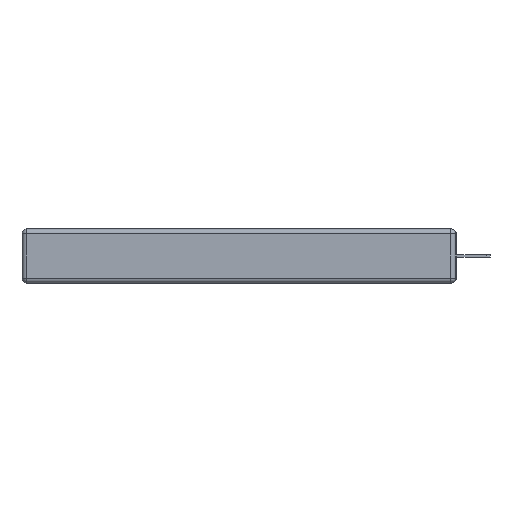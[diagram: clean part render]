
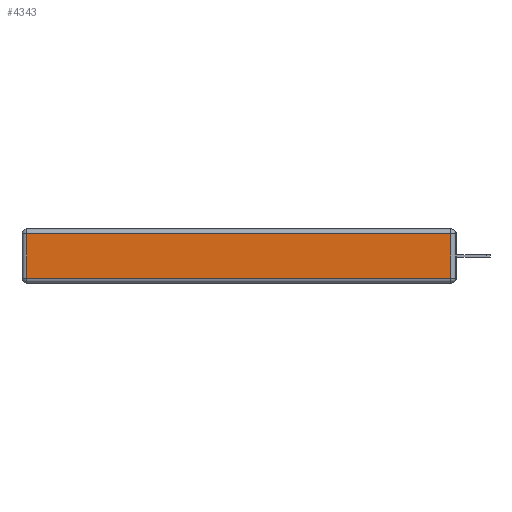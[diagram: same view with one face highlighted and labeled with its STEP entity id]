
A CAD part, left-side view. The second image highlights one B-rep face of the part: STEP entity #4343.
In plain terms, the highlighted planar face has unit normal (-1, 0, 0).
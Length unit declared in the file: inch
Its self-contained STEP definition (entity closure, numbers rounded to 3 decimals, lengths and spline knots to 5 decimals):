
#476 = ORIENTED_EDGE ( 'NONE', *, *, #2474, .T. ) ;
#554 = CARTESIAN_POINT ( 'NONE',  ( 0., 2.72, -0.313 ) ) ;
#595 = EDGE_CURVE ( 'NONE', #10657, #6561, #13023, .T. ) ;
#904 = EDGE_CURVE ( 'NONE', #5316, #4142, #4007, .T. ) ;
#1294 = VECTOR ( 'NONE', #12662, 39.37008 ) ;
#2042 = CARTESIAN_POINT ( 'NONE',  ( 0., 2.72, -0.343 ) ) ;
#2089 = DIRECTION ( 'NONE',  ( 0., 0., 1. ) ) ;
#2428 = CARTESIAN_POINT ( 'NONE',  ( 0., 0.03, -0.313 ) ) ;
#2474 = EDGE_CURVE ( 'NONE', #6561, #5316, #13754, .T. ) ;
#2563 = ORIENTED_EDGE ( 'NONE', *, *, #904, .T. ) ;
#3129 = PLANE ( 'NONE',  #13316 ) ;
#4007 = LINE ( 'NONE', #2042, #1294 ) ;
#4142 = VERTEX_POINT ( 'NONE', #554 ) ;
#4343 = ADVANCED_FACE ( 'NONE', ( #8448 ), #3129, .T. ) ;
#5254 = VECTOR ( 'NONE', #13088, 39.37008 ) ;
#5316 = VERTEX_POINT ( 'NONE', #9925 ) ;
#6561 = VERTEX_POINT ( 'NONE', #8897 ) ;
#6826 = ORIENTED_EDGE ( 'NONE', *, *, #10682, .T. ) ;
#7398 = CARTESIAN_POINT ( 'NONE',  ( 0., 0., -0.343 ) ) ;
#7810 = LINE ( 'NONE', #12065, #9044 ) ;
#8065 = VECTOR ( 'NONE', #8462, 39.37008 ) ;
#8448 = FACE_OUTER_BOUND ( 'NONE', #8768, .T. ) ;
#8462 = DIRECTION ( 'NONE',  ( 0., 1., 0. ) ) ;
#8768 = EDGE_LOOP ( 'NONE', ( #6826, #12038, #476, #2563 ) ) ;
#8897 = CARTESIAN_POINT ( 'NONE',  ( 0., 0.03, -0.03 ) ) ;
#8923 = DIRECTION ( 'NONE',  ( 0., -1., 0. ) ) ;
#9044 = VECTOR ( 'NONE', #8923, 39.37008 ) ;
#9438 = CARTESIAN_POINT ( 'NONE',  ( 0., 2.75, -0.03 ) ) ;
#9925 = CARTESIAN_POINT ( 'NONE',  ( 0., 2.72, -0.03 ) ) ;
#10657 = VERTEX_POINT ( 'NONE', #2428 ) ;
#10682 = EDGE_CURVE ( 'NONE', #4142, #10657, #7810, .T. ) ;
#10725 = CARTESIAN_POINT ( 'NONE',  ( 0., 0.03, -0.343 ) ) ;
#11657 = DIRECTION ( 'NONE',  ( -1., 0., 0. ) ) ;
#12038 = ORIENTED_EDGE ( 'NONE', *, *, #595, .T. ) ;
#12065 = CARTESIAN_POINT ( 'NONE',  ( 0., 0., -0.313 ) ) ;
#12662 = DIRECTION ( 'NONE',  ( 0., 0., -1. ) ) ;
#13023 = LINE ( 'NONE', #10725, #5254 ) ;
#13088 = DIRECTION ( 'NONE',  ( 0., 0., 1. ) ) ;
#13316 = AXIS2_PLACEMENT_3D ( 'NONE', #7398, #11657, #2089 ) ;
#13754 = LINE ( 'NONE', #9438, #8065 ) ;
